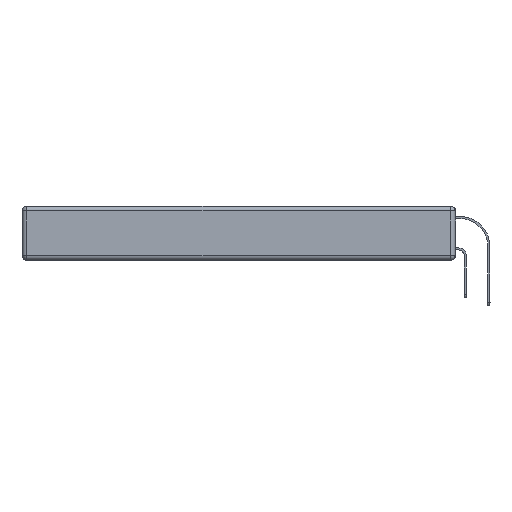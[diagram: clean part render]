
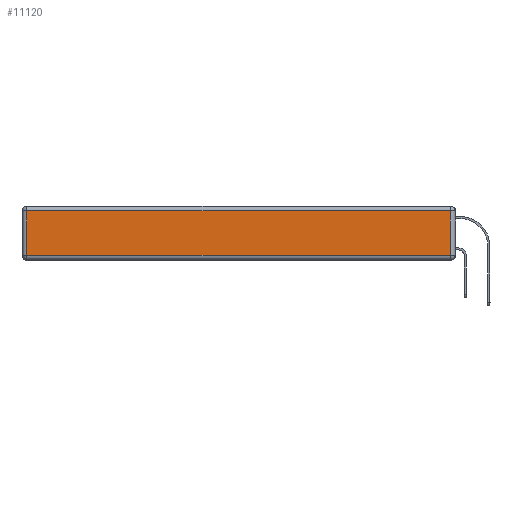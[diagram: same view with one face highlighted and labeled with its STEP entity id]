
A CAD part, left-side view. The second image highlights one B-rep face of the part: STEP entity #11120.
In plain terms, the highlighted planar face has unit normal (-1, 0, 0).
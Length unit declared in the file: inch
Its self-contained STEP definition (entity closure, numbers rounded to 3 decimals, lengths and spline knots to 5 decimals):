
#968 = CARTESIAN_POINT ( 'NONE',  ( 0., 0.03, -0.343 ) ) ;
#1203 = PLANE ( 'NONE',  #27023 ) ;
#1438 = CARTESIAN_POINT ( 'NONE',  ( 0., 0., -0.313 ) ) ;
#4330 = EDGE_CURVE ( 'NONE', #21076, #23604, #8823, .T. ) ;
#4497 = VECTOR ( 'NONE', #24419, 39.37008 ) ;
#4631 = VERTEX_POINT ( 'NONE', #11053 ) ;
#4807 = ORIENTED_EDGE ( 'NONE', *, *, #14430, .T. ) ;
#5596 = CARTESIAN_POINT ( 'NONE',  ( 0., 0., -0.343 ) ) ;
#6000 = CARTESIAN_POINT ( 'NONE',  ( 0., 2.72, -0.313 ) ) ;
#7584 = VERTEX_POINT ( 'NONE', #14719 ) ;
#8823 = LINE ( 'NONE', #26282, #15603 ) ;
#8854 = VECTOR ( 'NONE', #9535, 39.37008 ) ;
#9535 = DIRECTION ( 'NONE',  ( 0., 1., 0. ) ) ;
#10100 = DIRECTION ( 'NONE',  ( 0., 0., 1. ) ) ;
#11053 = CARTESIAN_POINT ( 'NONE',  ( 0., 0.03, -0.313 ) ) ;
#11120 = ADVANCED_FACE ( 'NONE', ( #24351 ), #1203, .T. ) ;
#13770 = CARTESIAN_POINT ( 'NONE',  ( 0., 2.75, -0.03 ) ) ;
#14151 = LINE ( 'NONE', #1438, #4497 ) ;
#14430 = EDGE_CURVE ( 'NONE', #7584, #21076, #22010, .T. ) ;
#14719 = CARTESIAN_POINT ( 'NONE',  ( 0., 0.03, -0.03 ) ) ;
#15324 = DIRECTION ( 'NONE',  ( 0., 0., 1. ) ) ;
#15495 = CARTESIAN_POINT ( 'NONE',  ( 0., 2.72, -0.03 ) ) ;
#15603 = VECTOR ( 'NONE', #21391, 39.37008 ) ;
#15819 = ORIENTED_EDGE ( 'NONE', *, *, #4330, .T. ) ;
#18625 = EDGE_CURVE ( 'NONE', #4631, #7584, #25721, .T. ) ;
#19330 = EDGE_LOOP ( 'NONE', ( #19973, #20383, #4807, #15819 ) ) ;
#19972 = DIRECTION ( 'NONE',  ( -1., 0., 0. ) ) ;
#19973 = ORIENTED_EDGE ( 'NONE', *, *, #20708, .T. ) ;
#20383 = ORIENTED_EDGE ( 'NONE', *, *, #18625, .T. ) ;
#20708 = EDGE_CURVE ( 'NONE', #23604, #4631, #14151, .T. ) ;
#21076 = VERTEX_POINT ( 'NONE', #15495 ) ;
#21391 = DIRECTION ( 'NONE',  ( 0., 0., -1. ) ) ;
#22010 = LINE ( 'NONE', #13770, #8854 ) ;
#22843 = VECTOR ( 'NONE', #15324, 39.37008 ) ;
#23604 = VERTEX_POINT ( 'NONE', #6000 ) ;
#24351 = FACE_OUTER_BOUND ( 'NONE', #19330, .T. ) ;
#24419 = DIRECTION ( 'NONE',  ( 0., -1., 0. ) ) ;
#25721 = LINE ( 'NONE', #968, #22843 ) ;
#26282 = CARTESIAN_POINT ( 'NONE',  ( 0., 2.72, -0.343 ) ) ;
#27023 = AXIS2_PLACEMENT_3D ( 'NONE', #5596, #19972, #10100 ) ;
